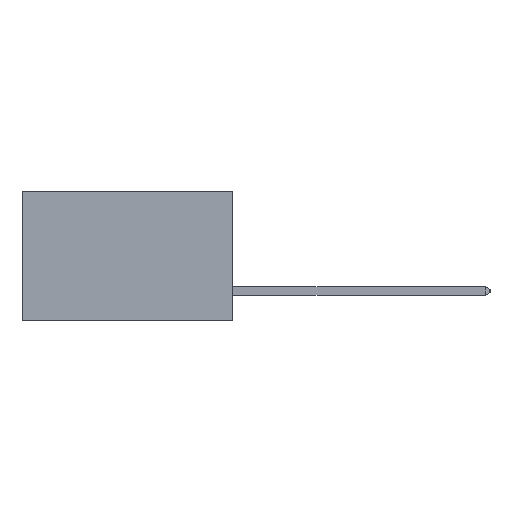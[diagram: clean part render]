
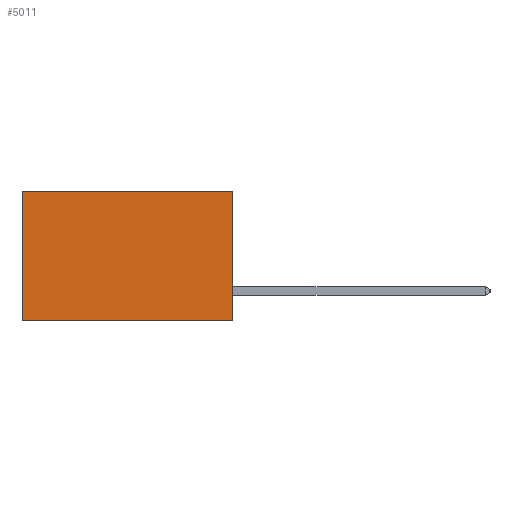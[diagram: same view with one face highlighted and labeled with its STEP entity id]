
A CAD part, left-side view. The second image highlights one B-rep face of the part: STEP entity #5011.
In plain terms, the highlighted planar face has unit normal (-1, 0, 0).
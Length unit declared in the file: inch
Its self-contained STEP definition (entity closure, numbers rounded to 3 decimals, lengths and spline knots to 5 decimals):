
#400 = EDGE_CURVE ( 'NONE', #8113, #22804, #12896, .T. ) ;
#1754 = VECTOR ( 'NONE', #21850, 39.37008 ) ;
#1882 = VECTOR ( 'NONE', #16765, 39.37008 ) ;
#2514 = CARTESIAN_POINT ( 'NONE',  ( 0.2875, 0., 0. ) ) ;
#3264 = VECTOR ( 'NONE', #3549, 39.37008 ) ;
#3509 = EDGE_CURVE ( 'NONE', #3737, #8113, #16450, .T. ) ;
#3549 = DIRECTION ( 'NONE',  ( 0., 1., 0. ) ) ;
#3737 = VERTEX_POINT ( 'NONE', #2514 ) ;
#3807 = ORIENTED_EDGE ( 'NONE', *, *, #3509, .T. ) ;
#4300 = CARTESIAN_POINT ( 'NONE',  ( 0.2875, 0., 0. ) ) ;
#4867 = FACE_OUTER_BOUND ( 'NONE', #10278, .T. ) ;
#5011 = ADVANCED_FACE ( 'NONE', ( #4867 ), #6964, .F. ) ;
#6502 = ORIENTED_EDGE ( 'NONE', *, *, #20621, .F. ) ;
#6787 = DIRECTION ( 'NONE',  ( 0., 0., -1. ) ) ;
#6809 = DIRECTION ( 'NONE',  ( 1., 0., 0. ) ) ;
#6964 = PLANE ( 'NONE',  #19921 ) ;
#7056 = CARTESIAN_POINT ( 'NONE',  ( 0.2875, 0., 0. ) ) ;
#8113 = VERTEX_POINT ( 'NONE', #13161 ) ;
#8519 = CARTESIAN_POINT ( 'NONE',  ( 0.2875, 0.6, -0.37 ) ) ;
#10278 = EDGE_LOOP ( 'NONE', ( #22097, #20496, #6502, #3807 ) ) ;
#11688 = CARTESIAN_POINT ( 'NONE',  ( 0.2875, 0., -0.37 ) ) ;
#12896 = LINE ( 'NONE', #21663, #22087 ) ;
#13161 = CARTESIAN_POINT ( 'NONE',  ( 0.2875, 0.6, 0. ) ) ;
#13922 = EDGE_CURVE ( 'NONE', #20089, #22804, #17358, .T. ) ;
#14924 = CARTESIAN_POINT ( 'NONE',  ( 0.2875, 0., 0. ) ) ;
#15986 = LINE ( 'NONE', #14924, #1882 ) ;
#16450 = LINE ( 'NONE', #4300, #1754 ) ;
#16765 = DIRECTION ( 'NONE',  ( 0., 0., -1. ) ) ;
#17358 = LINE ( 'NONE', #19995, #3264 ) ;
#17980 = DIRECTION ( 'NONE',  ( 0., 0., -1. ) ) ;
#19921 = AXIS2_PLACEMENT_3D ( 'NONE', #7056, #6809, #6787 ) ;
#19995 = CARTESIAN_POINT ( 'NONE',  ( 0.2875, 0., -0.37 ) ) ;
#20089 = VERTEX_POINT ( 'NONE', #11688 ) ;
#20496 = ORIENTED_EDGE ( 'NONE', *, *, #13922, .F. ) ;
#20621 = EDGE_CURVE ( 'NONE', #3737, #20089, #15986, .T. ) ;
#21663 = CARTESIAN_POINT ( 'NONE',  ( 0.2875, 0.6, 0. ) ) ;
#21850 = DIRECTION ( 'NONE',  ( 0., 1., 0. ) ) ;
#22087 = VECTOR ( 'NONE', #17980, 39.37008 ) ;
#22097 = ORIENTED_EDGE ( 'NONE', *, *, #400, .T. ) ;
#22804 = VERTEX_POINT ( 'NONE', #8519 ) ;
